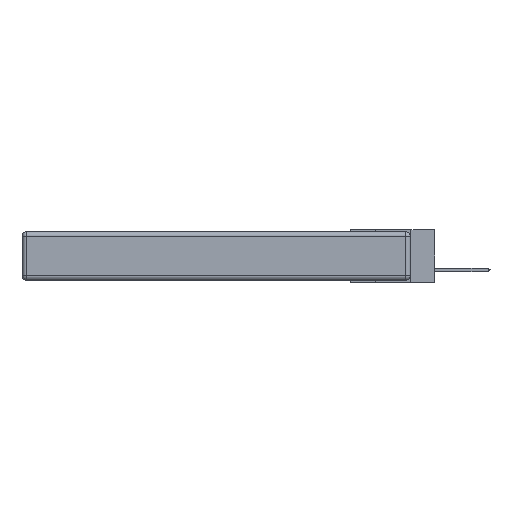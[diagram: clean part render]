
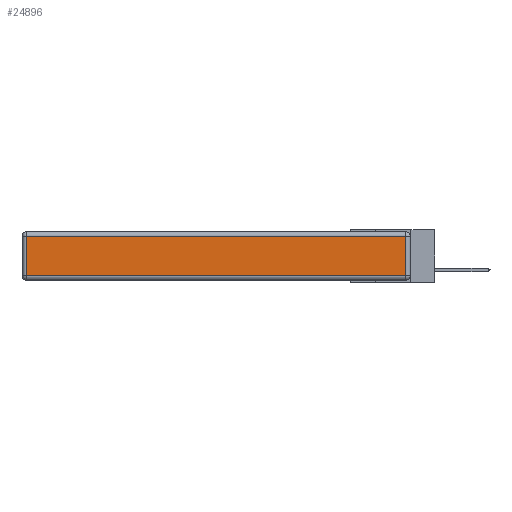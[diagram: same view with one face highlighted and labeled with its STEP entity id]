
A CAD part, left-side view. The second image highlights one B-rep face of the part: STEP entity #24896.
In plain terms, the highlighted planar face has unit normal (-1, 0, 0).
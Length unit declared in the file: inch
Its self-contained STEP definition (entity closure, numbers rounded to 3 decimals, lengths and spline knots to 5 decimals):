
#1088 = EDGE_CURVE ( 'NONE', #7208, #28391, #8225, .T. ) ;
#1319 = CARTESIAN_POINT ( 'NONE',  ( 0., 2.72, -0.03 ) ) ;
#1948 = VECTOR ( 'NONE', #19120, 39.37008 ) ;
#2373 = DIRECTION ( 'NONE',  ( 0., 1., 0. ) ) ;
#3835 = ORIENTED_EDGE ( 'NONE', *, *, #18500, .T. ) ;
#4156 = ORIENTED_EDGE ( 'NONE', *, *, #7504, .T. ) ;
#5518 = DIRECTION ( 'NONE',  ( 0., 0., 1. ) ) ;
#5624 = CARTESIAN_POINT ( 'NONE',  ( 0., 0.03, -0.343 ) ) ;
#7208 = VERTEX_POINT ( 'NONE', #1319 ) ;
#7504 = EDGE_CURVE ( 'NONE', #18414, #7208, #9092, .T. ) ;
#8225 = LINE ( 'NONE', #8745, #22851 ) ;
#8745 = CARTESIAN_POINT ( 'NONE',  ( 0., 2.72, -0.343 ) ) ;
#9092 = LINE ( 'NONE', #14510, #18027 ) ;
#10725 = DIRECTION ( 'NONE',  ( 0., 0., -1. ) ) ;
#11676 = EDGE_CURVE ( 'NONE', #22028, #18414, #12281, .T. ) ;
#12281 = LINE ( 'NONE', #5624, #28805 ) ;
#12484 = DIRECTION ( 'NONE',  ( -1., 0., 0. ) ) ;
#12666 = CARTESIAN_POINT ( 'NONE',  ( 0., 0.03, -0.313 ) ) ;
#14510 = CARTESIAN_POINT ( 'NONE',  ( 0., 2.75, -0.03 ) ) ;
#18027 = VECTOR ( 'NONE', #2373, 39.37008 ) ;
#18414 = VERTEX_POINT ( 'NONE', #20202 ) ;
#18500 = EDGE_CURVE ( 'NONE', #28391, #22028, #24407, .T. ) ;
#19097 = ORIENTED_EDGE ( 'NONE', *, *, #1088, .T. ) ;
#19120 = DIRECTION ( 'NONE',  ( 0., -1., 0. ) ) ;
#20202 = CARTESIAN_POINT ( 'NONE',  ( 0., 0.03, -0.03 ) ) ;
#22028 = VERTEX_POINT ( 'NONE', #12666 ) ;
#22037 = DIRECTION ( 'NONE',  ( 0., 0., 1. ) ) ;
#22851 = VECTOR ( 'NONE', #10725, 39.37008 ) ;
#24407 = LINE ( 'NONE', #30873, #1948 ) ;
#24896 = ADVANCED_FACE ( 'NONE', ( #25106 ), #26441, .T. ) ;
#25106 = FACE_OUTER_BOUND ( 'NONE', #26030, .T. ) ;
#25116 = ORIENTED_EDGE ( 'NONE', *, *, #11676, .T. ) ;
#26030 = EDGE_LOOP ( 'NONE', ( #3835, #25116, #4156, #19097 ) ) ;
#26441 = PLANE ( 'NONE',  #27505 ) ;
#27505 = AXIS2_PLACEMENT_3D ( 'NONE', #28833, #12484, #22037 ) ;
#28391 = VERTEX_POINT ( 'NONE', #29255 ) ;
#28805 = VECTOR ( 'NONE', #5518, 39.37008 ) ;
#28833 = CARTESIAN_POINT ( 'NONE',  ( 0., 0., -0.343 ) ) ;
#29255 = CARTESIAN_POINT ( 'NONE',  ( 0., 2.72, -0.313 ) ) ;
#30873 = CARTESIAN_POINT ( 'NONE',  ( 0., 0., -0.313 ) ) ;
